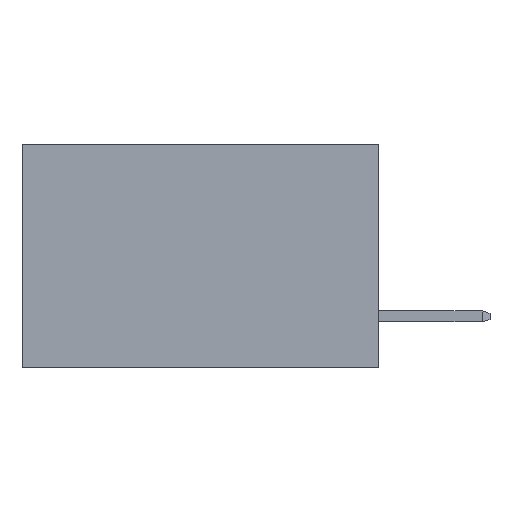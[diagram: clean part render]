
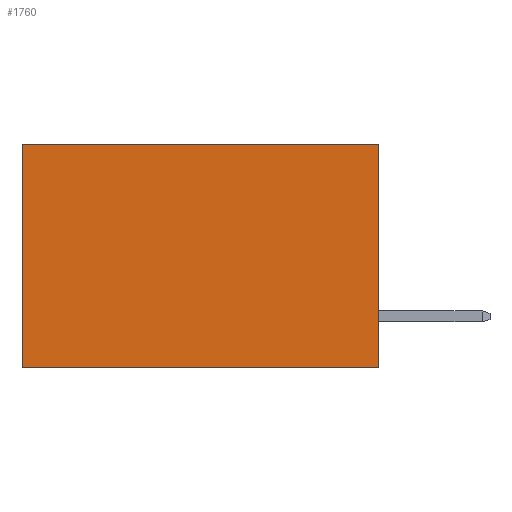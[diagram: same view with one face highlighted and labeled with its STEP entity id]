
A CAD part, left-side view. The second image highlights one B-rep face of the part: STEP entity #1760.
In plain terms, the highlighted planar face has unit normal (-1, 0, 0).
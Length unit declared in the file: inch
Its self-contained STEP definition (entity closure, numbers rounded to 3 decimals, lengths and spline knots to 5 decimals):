
#609 = CARTESIAN_POINT ( 'NONE',  ( 0.277, 0.59, 0. ) ) ;
#899 = VECTOR ( 'NONE', #6448, 39.37008 ) ;
#909 = VERTEX_POINT ( 'NONE', #609 ) ;
#1134 = LINE ( 'NONE', #6506, #899 ) ;
#1362 = VECTOR ( 'NONE', #6686, 39.37008 ) ;
#1588 = VECTOR ( 'NONE', #7343, 39.37008 ) ;
#1619 = CARTESIAN_POINT ( 'NONE',  ( 0.277, 0.59, -0.37 ) ) ;
#1760 = ADVANCED_FACE ( 'NONE', ( #5900 ), #5972, .F. ) ;
#2072 = LINE ( 'NONE', #6216, #8092 ) ;
#2157 = VERTEX_POINT ( 'NONE', #1619 ) ;
#2447 = EDGE_CURVE ( 'NONE', #7781, #2157, #2072, .T. ) ;
#2730 = EDGE_LOOP ( 'NONE', ( #5039, #5148, #5229, #5433 ) ) ;
#2886 = CARTESIAN_POINT ( 'NONE',  ( 0.277, 0., 0. ) ) ;
#3202 = LINE ( 'NONE', #7279, #1362 ) ;
#3675 = CARTESIAN_POINT ( 'NONE',  ( 0.277, 0., -0.37 ) ) ;
#4693 = VERTEX_POINT ( 'NONE', #2886 ) ;
#5039 = ORIENTED_EDGE ( 'NONE', *, *, #8238, .T. ) ;
#5148 = ORIENTED_EDGE ( 'NONE', *, *, #2447, .F. ) ;
#5162 = LINE ( 'NONE', #7335, #1588 ) ;
#5229 = ORIENTED_EDGE ( 'NONE', *, *, #7660, .F. ) ;
#5433 = ORIENTED_EDGE ( 'NONE', *, *, #8200, .T. ) ;
#5549 = CARTESIAN_POINT ( 'NONE',  ( 0.277, 0., -0.37 ) ) ;
#5900 = FACE_OUTER_BOUND ( 'NONE', #2730, .T. ) ;
#5972 = PLANE ( 'NONE',  #7129 ) ;
#6216 = CARTESIAN_POINT ( 'NONE',  ( 0.277, 0., -0.37 ) ) ;
#6448 = DIRECTION ( 'NONE',  ( 0., 0., -1. ) ) ;
#6506 = CARTESIAN_POINT ( 'NONE',  ( 0.277, 0.59, -0.37 ) ) ;
#6686 = DIRECTION ( 'NONE',  ( 0., 1., 0. ) ) ;
#6739 = DIRECTION ( 'NONE',  ( 0., 0., -1. ) ) ;
#6917 = DIRECTION ( 'NONE',  ( 1., 0., 0. ) ) ;
#7129 = AXIS2_PLACEMENT_3D ( 'NONE', #5549, #6917, #6739 ) ;
#7141 = DIRECTION ( 'NONE',  ( 0., 1., 0. ) ) ;
#7279 = CARTESIAN_POINT ( 'NONE',  ( 0.277, 0., 0. ) ) ;
#7335 = CARTESIAN_POINT ( 'NONE',  ( 0.277, 0., -0.37 ) ) ;
#7343 = DIRECTION ( 'NONE',  ( 0., 0., -1. ) ) ;
#7660 = EDGE_CURVE ( 'NONE', #4693, #7781, #5162, .T. ) ;
#7781 = VERTEX_POINT ( 'NONE', #3675 ) ;
#8092 = VECTOR ( 'NONE', #7141, 39.37008 ) ;
#8200 = EDGE_CURVE ( 'NONE', #4693, #909, #3202, .T. ) ;
#8238 = EDGE_CURVE ( 'NONE', #909, #2157, #1134, .T. ) ;
